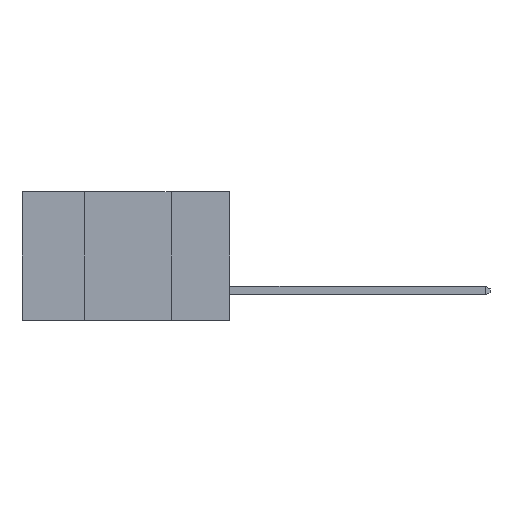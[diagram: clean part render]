
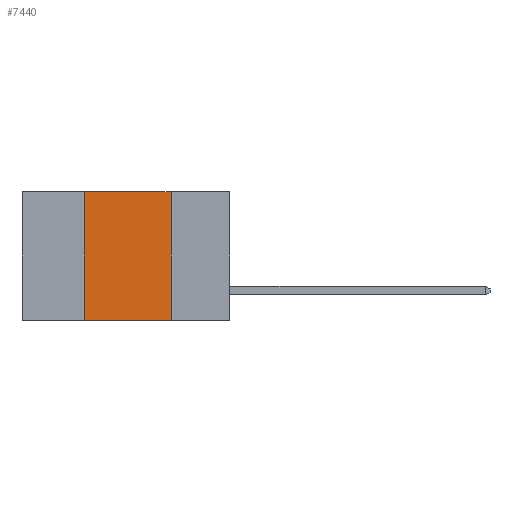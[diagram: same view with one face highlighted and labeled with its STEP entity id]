
A CAD part, left-side view. The second image highlights one B-rep face of the part: STEP entity #7440.
In plain terms, the highlighted planar face has unit normal (-1, 0, 0).
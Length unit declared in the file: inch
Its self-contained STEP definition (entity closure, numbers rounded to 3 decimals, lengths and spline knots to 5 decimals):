
#512 = ORIENTED_EDGE ( 'NONE', *, *, #1080, .F. ) ;
#735 = EDGE_LOOP ( 'NONE', ( #3548, #512, #5695, #11900 ) ) ;
#1080 = EDGE_CURVE ( 'NONE', #8360, #9262, #9630, .T. ) ;
#1478 = CARTESIAN_POINT ( 'NONE',  ( 0., 0.17, 0. ) ) ;
#1554 = DIRECTION ( 'NONE',  ( 0., 0., -1. ) ) ;
#2032 = CARTESIAN_POINT ( 'NONE',  ( 0., 0.17, -0.37 ) ) ;
#2067 = DIRECTION ( 'NONE',  ( 0., -1., 0. ) ) ;
#2566 = DIRECTION ( 'NONE',  ( 0., 0., 1. ) ) ;
#2847 = VECTOR ( 'NONE', #1554, 39.37008 ) ;
#2933 = LINE ( 'NONE', #7836, #5434 ) ;
#3184 = LINE ( 'NONE', #11374, #8241 ) ;
#3187 = EDGE_CURVE ( 'NONE', #9262, #3534, #11313, .T. ) ;
#3534 = VERTEX_POINT ( 'NONE', #2032 ) ;
#3548 = ORIENTED_EDGE ( 'NONE', *, *, #3187, .F. ) ;
#3641 = VERTEX_POINT ( 'NONE', #9908 ) ;
#4069 = VECTOR ( 'NONE', #2067, 39.37008 ) ;
#5434 = VECTOR ( 'NONE', #6282, 39.37008 ) ;
#5695 = ORIENTED_EDGE ( 'NONE', *, *, #12539, .F. ) ;
#6000 = DIRECTION ( 'NONE',  ( 0., 0., -1. ) ) ;
#6282 = DIRECTION ( 'NONE',  ( 0., -1., 0. ) ) ;
#6304 = EDGE_CURVE ( 'NONE', #3641, #3534, #2933, .T. ) ;
#7238 = CARTESIAN_POINT ( 'NONE',  ( 0., 0.17, 0. ) ) ;
#7440 = ADVANCED_FACE ( 'NONE', ( #9481 ), #10588, .F. ) ;
#7727 = DIRECTION ( 'NONE',  ( 1., 0., 0. ) ) ;
#7836 = CARTESIAN_POINT ( 'NONE',  ( 0., 0.6, -0.37 ) ) ;
#8241 = VECTOR ( 'NONE', #2566, 39.37008 ) ;
#8360 = VERTEX_POINT ( 'NONE', #8528 ) ;
#8528 = CARTESIAN_POINT ( 'NONE',  ( 0., 0.42, 0. ) ) ;
#9262 = VERTEX_POINT ( 'NONE', #7238 ) ;
#9481 = FACE_OUTER_BOUND ( 'NONE', #735, .T. ) ;
#9630 = LINE ( 'NONE', #11761, #4069 ) ;
#9687 = AXIS2_PLACEMENT_3D ( 'NONE', #11633, #7727, #6000 ) ;
#9908 = CARTESIAN_POINT ( 'NONE',  ( 0., 0.42, -0.37 ) ) ;
#10588 = PLANE ( 'NONE',  #9687 ) ;
#11313 = LINE ( 'NONE', #1478, #2847 ) ;
#11374 = CARTESIAN_POINT ( 'NONE',  ( 0., 0.42, 0. ) ) ;
#11633 = CARTESIAN_POINT ( 'NONE',  ( 0., 0.6, 0. ) ) ;
#11761 = CARTESIAN_POINT ( 'NONE',  ( 0., 0.6, 0. ) ) ;
#11900 = ORIENTED_EDGE ( 'NONE', *, *, #6304, .T. ) ;
#12539 = EDGE_CURVE ( 'NONE', #3641, #8360, #3184, .T. ) ;
